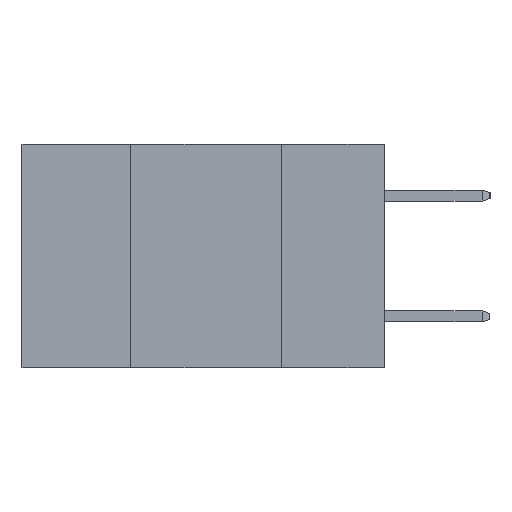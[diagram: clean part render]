
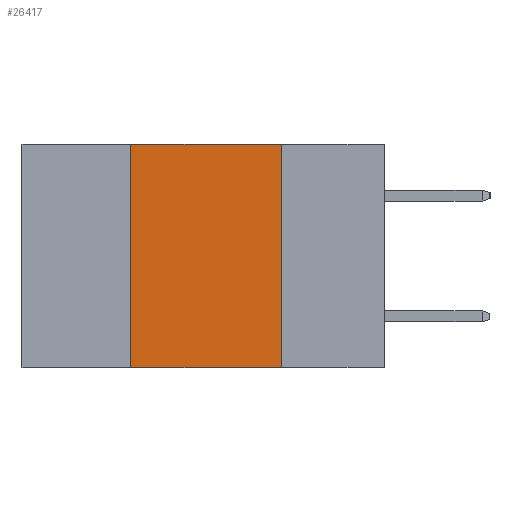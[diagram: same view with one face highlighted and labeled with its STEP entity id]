
A CAD part, left-side view. The second image highlights one B-rep face of the part: STEP entity #26417.
In plain terms, the highlighted planar face has unit normal (-1, 0, 0).
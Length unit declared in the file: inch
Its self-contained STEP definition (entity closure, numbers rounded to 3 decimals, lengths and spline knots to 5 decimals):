
#974 = CARTESIAN_POINT ( 'NONE',  ( 0., 0.42, 0. ) ) ;
#1975 = VERTEX_POINT ( 'NONE', #974 ) ;
#2350 = CARTESIAN_POINT ( 'NONE',  ( 0., 0.6, -0.37 ) ) ;
#3171 = CARTESIAN_POINT ( 'NONE',  ( 0., 0.6, 0. ) ) ;
#5418 = DIRECTION ( 'NONE',  ( 1., 0., 0. ) ) ;
#5859 = DIRECTION ( 'NONE',  ( 0., 0., 1. ) ) ;
#5948 = AXIS2_PLACEMENT_3D ( 'NONE', #23974, #5418, #13680 ) ;
#6959 = VERTEX_POINT ( 'NONE', #13331 ) ;
#7783 = VERTEX_POINT ( 'NONE', #23310 ) ;
#7813 = EDGE_LOOP ( 'NONE', ( #20833, #23954, #26414, #17425 ) ) ;
#8872 = EDGE_CURVE ( 'NONE', #9832, #1975, #18199, .T. ) ;
#8924 = DIRECTION ( 'NONE',  ( 0., 0., -1. ) ) ;
#9404 = LINE ( 'NONE', #3171, #20660 ) ;
#9502 = VECTOR ( 'NONE', #5859, 39.37008 ) ;
#9630 = EDGE_CURVE ( 'NONE', #7783, #6959, #19220, .T. ) ;
#9832 = VERTEX_POINT ( 'NONE', #16377 ) ;
#11423 = DIRECTION ( 'NONE',  ( 0., -1., 0. ) ) ;
#11887 = EDGE_CURVE ( 'NONE', #1975, #7783, #9404, .T. ) ;
#13250 = CARTESIAN_POINT ( 'NONE',  ( 0., 0.17, -0.37 ) ) ;
#13331 = CARTESIAN_POINT ( 'NONE',  ( 0., 0.17, -0.37 ) ) ;
#13680 = DIRECTION ( 'NONE',  ( 0., 0., -1. ) ) ;
#15725 = FACE_OUTER_BOUND ( 'NONE', #7813, .T. ) ;
#16377 = CARTESIAN_POINT ( 'NONE',  ( 0., 0.42, -0.37 ) ) ;
#17006 = VECTOR ( 'NONE', #17904, 39.37008 ) ;
#17425 = ORIENTED_EDGE ( 'NONE', *, *, #18333, .T. ) ;
#17904 = DIRECTION ( 'NONE',  ( 0., -1., 0. ) ) ;
#18199 = LINE ( 'NONE', #24413, #9502 ) ;
#18333 = EDGE_CURVE ( 'NONE', #9832, #6959, #20897, .T. ) ;
#19220 = LINE ( 'NONE', #13250, #24968 ) ;
#20191 = PLANE ( 'NONE',  #5948 ) ;
#20660 = VECTOR ( 'NONE', #11423, 39.37008 ) ;
#20833 = ORIENTED_EDGE ( 'NONE', *, *, #9630, .F. ) ;
#20897 = LINE ( 'NONE', #2350, #17006 ) ;
#23310 = CARTESIAN_POINT ( 'NONE',  ( 0., 0.17, 0. ) ) ;
#23954 = ORIENTED_EDGE ( 'NONE', *, *, #11887, .F. ) ;
#23974 = CARTESIAN_POINT ( 'NONE',  ( 0., 0.6, 0. ) ) ;
#24413 = CARTESIAN_POINT ( 'NONE',  ( 0., 0.42, -0.37 ) ) ;
#24968 = VECTOR ( 'NONE', #8924, 39.37008 ) ;
#26414 = ORIENTED_EDGE ( 'NONE', *, *, #8872, .F. ) ;
#26417 = ADVANCED_FACE ( 'NONE', ( #15725 ), #20191, .F. ) ;
